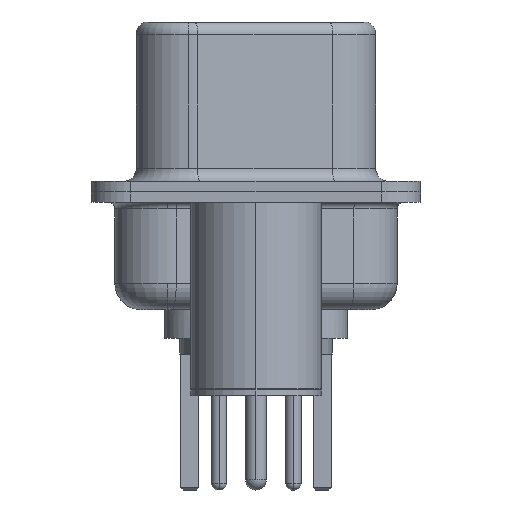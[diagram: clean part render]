
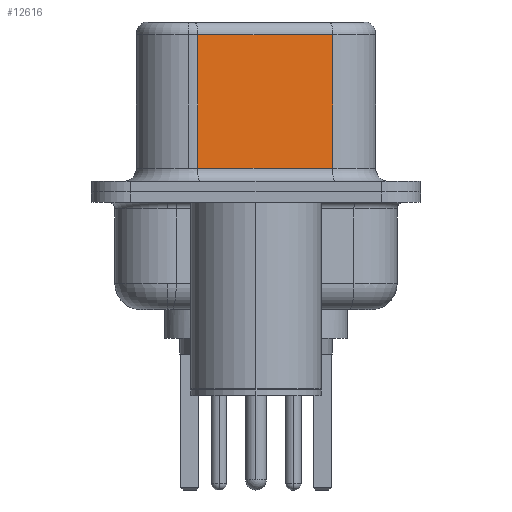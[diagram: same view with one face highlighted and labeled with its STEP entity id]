
A CAD part, left-side view. The second image highlights one B-rep face of the part: STEP entity #12616.
In plain terms, the highlighted planar face has unit normal (-0.985, -0.174, 0).
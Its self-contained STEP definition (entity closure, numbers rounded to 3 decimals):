
#841 = DIRECTION ( 'NONE',  ( -0.174, 0.985, 0. ) ) ;
#1308 = EDGE_CURVE ( 'NONE', #11669, #1945, #19730, .T. ) ;
#1582 = VERTEX_POINT ( 'NONE', #4346 ) ;
#1945 = VERTEX_POINT ( 'NONE', #20999 ) ;
#2457 = ORIENTED_EDGE ( 'NONE', *, *, #10957, .T. ) ;
#3615 = CARTESIAN_POINT ( 'NONE',  ( 4.585, -2.927, 0.9 ) ) ;
#3736 = ORIENTED_EDGE ( 'NONE', *, *, #13850, .F. ) ;
#4266 = VECTOR ( 'NONE', #6382, 1000. ) ;
#4346 = CARTESIAN_POINT ( 'NONE',  ( 3.675, 2.233, 6.02 ) ) ;
#4733 = VERTEX_POINT ( 'NONE', #21108 ) ;
#4884 = LINE ( 'NONE', #18237, #19385 ) ;
#6382 = DIRECTION ( 'NONE',  ( -0.174, 0.985, 0. ) ) ;
#6421 = ORIENTED_EDGE ( 'NONE', *, *, #1308, .T. ) ;
#7022 = FACE_OUTER_BOUND ( 'NONE', #16272, .T. ) ;
#8539 = CARTESIAN_POINT ( 'NONE',  ( 4.585, -2.927, 6.52 ) ) ;
#9670 = DIRECTION ( 'NONE',  ( 0., 0., -1. ) ) ;
#10957 = EDGE_CURVE ( 'NONE', #1582, #11669, #4884, .T. ) ;
#11322 = VECTOR ( 'NONE', #20991, 1000. ) ;
#11603 = CARTESIAN_POINT ( 'NONE',  ( 4.585, -2.927, 6.02 ) ) ;
#11669 = VERTEX_POINT ( 'NONE', #13056 ) ;
#12257 = LINE ( 'NONE', #11603, #4266 ) ;
#12616 = ADVANCED_FACE ( 'NONE', ( #7022 ), #16360, .F. ) ;
#13056 = CARTESIAN_POINT ( 'NONE',  ( 3.675, 2.233, 0.9 ) ) ;
#13850 = EDGE_CURVE ( 'NONE', #4733, #1945, #16021, .T. ) ;
#15225 = VECTOR ( 'NONE', #20688, 1000. ) ;
#16021 = LINE ( 'NONE', #8539, #15225 ) ;
#16272 = EDGE_LOOP ( 'NONE', ( #3736, #18292, #2457, #6421 ) ) ;
#16360 = PLANE ( 'NONE',  #16508 ) ;
#16508 = AXIS2_PLACEMENT_3D ( 'NONE', #21804, #19965, #841 ) ;
#18237 = CARTESIAN_POINT ( 'NONE',  ( 3.675, 2.233, 6.52 ) ) ;
#18292 = ORIENTED_EDGE ( 'NONE', *, *, #19550, .T. ) ;
#19385 = VECTOR ( 'NONE', #9670, 1000. ) ;
#19550 = EDGE_CURVE ( 'NONE', #4733, #1582, #12257, .T. ) ;
#19730 = LINE ( 'NONE', #3615, #11322 ) ;
#19965 = DIRECTION ( 'NONE',  ( 0.985, 0.174, 0. ) ) ;
#20688 = DIRECTION ( 'NONE',  ( 0., 0., -1. ) ) ;
#20991 = DIRECTION ( 'NONE',  ( 0.174, -0.985, 0. ) ) ;
#20999 = CARTESIAN_POINT ( 'NONE',  ( 4.585, -2.927, 0.9 ) ) ;
#21108 = CARTESIAN_POINT ( 'NONE',  ( 4.585, -2.927, 6.02 ) ) ;
#21804 = CARTESIAN_POINT ( 'NONE',  ( 4.585, -2.927, 6.52 ) ) ;
